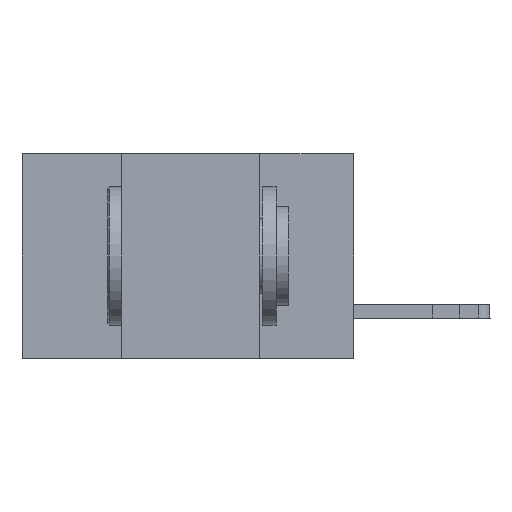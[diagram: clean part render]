
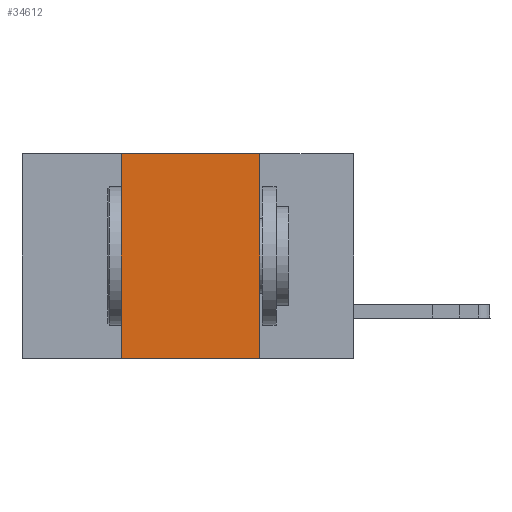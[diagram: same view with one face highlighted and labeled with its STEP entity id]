
A CAD part, left-side view. The second image highlights one B-rep face of the part: STEP entity #34612.
In plain terms, the highlighted planar face has unit normal (-1, 0, 0).
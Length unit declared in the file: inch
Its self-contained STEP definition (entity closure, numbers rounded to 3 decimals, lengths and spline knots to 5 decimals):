
#409 = EDGE_CURVE ( 'NONE', #19668, #6638, #17897, .T. ) ;
#4363 = LINE ( 'NONE', #30714, #38855 ) ;
#5116 = CARTESIAN_POINT ( 'NONE',  ( 0., 0.6, -0.37 ) ) ;
#5465 = VERTEX_POINT ( 'NONE', #28590 ) ;
#6638 = VERTEX_POINT ( 'NONE', #29051 ) ;
#6705 = CARTESIAN_POINT ( 'NONE',  ( 0., 0.42, -0.37 ) ) ;
#8307 = AXIS2_PLACEMENT_3D ( 'NONE', #9124, #39116, #30237 ) ;
#9124 = CARTESIAN_POINT ( 'NONE',  ( 0., 0.6, 0. ) ) ;
#9723 = DIRECTION ( 'NONE',  ( 0., 0., -1. ) ) ;
#12795 = ORIENTED_EDGE ( 'NONE', *, *, #409, .F. ) ;
#13091 = LINE ( 'NONE', #14864, #29173 ) ;
#14511 = ORIENTED_EDGE ( 'NONE', *, *, #23232, .T. ) ;
#14864 = CARTESIAN_POINT ( 'NONE',  ( 0., 0.6, 0. ) ) ;
#15052 = PLANE ( 'NONE',  #8307 ) ;
#17897 = LINE ( 'NONE', #21857, #27768 ) ;
#19624 = LINE ( 'NONE', #5116, #28559 ) ;
#19668 = VERTEX_POINT ( 'NONE', #6705 ) ;
#20676 = DIRECTION ( 'NONE',  ( 0., -1., 0. ) ) ;
#21300 = CARTESIAN_POINT ( 'NONE',  ( 0., 0.17, -0.37 ) ) ;
#21614 = EDGE_CURVE ( 'NONE', #6638, #5465, #13091, .T. ) ;
#21857 = CARTESIAN_POINT ( 'NONE',  ( 0., 0.42, 0. ) ) ;
#23232 = EDGE_CURVE ( 'NONE', #19668, #35995, #19624, .T. ) ;
#24443 = FACE_OUTER_BOUND ( 'NONE', #37578, .T. ) ;
#25258 = DIRECTION ( 'NONE',  ( 0., -1., 0. ) ) ;
#26590 = EDGE_CURVE ( 'NONE', #5465, #35995, #4363, .T. ) ;
#27768 = VECTOR ( 'NONE', #33845, 39.37008 ) ;
#28559 = VECTOR ( 'NONE', #25258, 39.37008 ) ;
#28590 = CARTESIAN_POINT ( 'NONE',  ( 0., 0.17, 0. ) ) ;
#29051 = CARTESIAN_POINT ( 'NONE',  ( 0., 0.42, 0. ) ) ;
#29173 = VECTOR ( 'NONE', #20676, 39.37008 ) ;
#30184 = ORIENTED_EDGE ( 'NONE', *, *, #26590, .F. ) ;
#30237 = DIRECTION ( 'NONE',  ( 0., 0., -1. ) ) ;
#30714 = CARTESIAN_POINT ( 'NONE',  ( 0., 0.17, 0. ) ) ;
#33686 = ORIENTED_EDGE ( 'NONE', *, *, #21614, .F. ) ;
#33845 = DIRECTION ( 'NONE',  ( 0., 0., 1. ) ) ;
#34612 = ADVANCED_FACE ( 'NONE', ( #24443 ), #15052, .F. ) ;
#35995 = VERTEX_POINT ( 'NONE', #21300 ) ;
#37578 = EDGE_LOOP ( 'NONE', ( #30184, #33686, #12795, #14511 ) ) ;
#38855 = VECTOR ( 'NONE', #9723, 39.37008 ) ;
#39116 = DIRECTION ( 'NONE',  ( 1., 0., 0. ) ) ;
